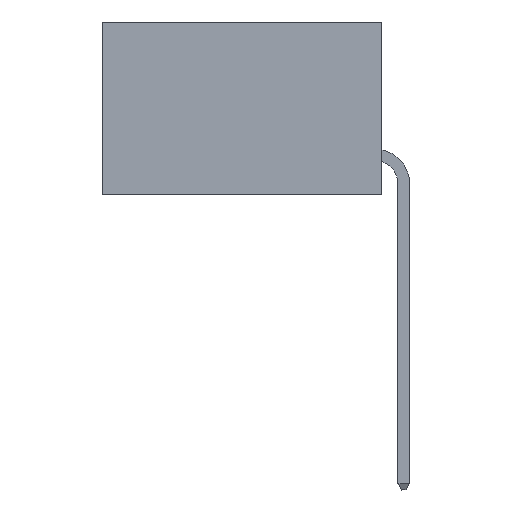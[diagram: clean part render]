
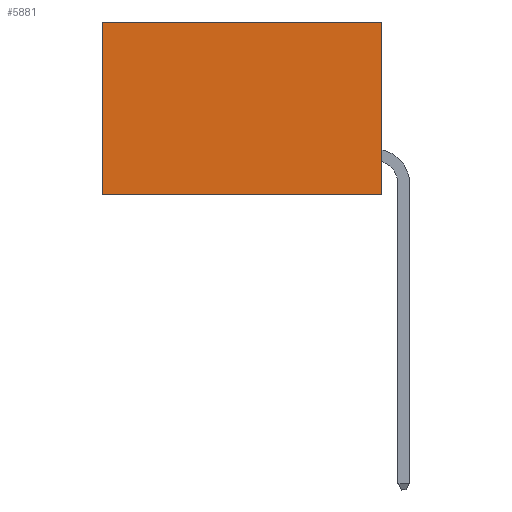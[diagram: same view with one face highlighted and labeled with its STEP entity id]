
A CAD part, left-side view. The second image highlights one B-rep face of the part: STEP entity #5881.
In plain terms, the highlighted planar face has unit normal (-1, 0, 0).
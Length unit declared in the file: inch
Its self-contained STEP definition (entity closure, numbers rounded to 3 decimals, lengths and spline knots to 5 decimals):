
#321 = EDGE_CURVE ( 'NONE', #15729, #2210, #14465, .T. ) ;
#1019 = VERTEX_POINT ( 'NONE', #22329 ) ;
#1737 = CARTESIAN_POINT ( 'NONE',  ( 0.2875, 0.6, -0.37 ) ) ;
#2210 = VERTEX_POINT ( 'NONE', #9588 ) ;
#4248 = EDGE_CURVE ( 'NONE', #2210, #4599, #11331, .T. ) ;
#4437 = PLANE ( 'NONE',  #33246 ) ;
#4599 = VERTEX_POINT ( 'NONE', #1737 ) ;
#4905 = VECTOR ( 'NONE', #11310, 39.37008 ) ;
#5881 = ADVANCED_FACE ( 'NONE', ( #37400 ), #4437, .F. ) ;
#7510 = DIRECTION ( 'NONE',  ( 1., 0., 0. ) ) ;
#7844 = VECTOR ( 'NONE', #12053, 39.37008 ) ;
#9588 = CARTESIAN_POINT ( 'NONE',  ( 0.2875, 0., -0.37 ) ) ;
#10782 = CARTESIAN_POINT ( 'NONE',  ( 0.2875, 0., 0. ) ) ;
#10983 = CARTESIAN_POINT ( 'NONE',  ( 0.2875, 0.6, 0. ) ) ;
#11310 = DIRECTION ( 'NONE',  ( 0., 1., 0. ) ) ;
#11331 = LINE ( 'NONE', #11595, #25569 ) ;
#11595 = CARTESIAN_POINT ( 'NONE',  ( 0.2875, 0., -0.37 ) ) ;
#12053 = DIRECTION ( 'NONE',  ( 0., 0., -1. ) ) ;
#14465 = LINE ( 'NONE', #30299, #7844 ) ;
#14658 = DIRECTION ( 'NONE',  ( 0., 1., 0. ) ) ;
#15729 = VERTEX_POINT ( 'NONE', #35232 ) ;
#16946 = DIRECTION ( 'NONE',  ( 0., 0., -1. ) ) ;
#18547 = ORIENTED_EDGE ( 'NONE', *, *, #22920, .T. ) ;
#19754 = CARTESIAN_POINT ( 'NONE',  ( 0.2875, 0., 0. ) ) ;
#22329 = CARTESIAN_POINT ( 'NONE',  ( 0.2875, 0.6, 0. ) ) ;
#22920 = EDGE_CURVE ( 'NONE', #1019, #4599, #33536, .T. ) ;
#23930 = LINE ( 'NONE', #10782, #4905 ) ;
#25569 = VECTOR ( 'NONE', #14658, 39.37008 ) ;
#29267 = ORIENTED_EDGE ( 'NONE', *, *, #4248, .F. ) ;
#30299 = CARTESIAN_POINT ( 'NONE',  ( 0.2875, 0., 0. ) ) ;
#32159 = DIRECTION ( 'NONE',  ( 0., 0., -1. ) ) ;
#32583 = VECTOR ( 'NONE', #32159, 39.37008 ) ;
#33246 = AXIS2_PLACEMENT_3D ( 'NONE', #19754, #7510, #16946 ) ;
#33536 = LINE ( 'NONE', #10983, #32583 ) ;
#34425 = ORIENTED_EDGE ( 'NONE', *, *, #321, .F. ) ;
#34855 = EDGE_LOOP ( 'NONE', ( #18547, #29267, #34425, #36736 ) ) ;
#35232 = CARTESIAN_POINT ( 'NONE',  ( 0.2875, 0., 0. ) ) ;
#36736 = ORIENTED_EDGE ( 'NONE', *, *, #38510, .T. ) ;
#37400 = FACE_OUTER_BOUND ( 'NONE', #34855, .T. ) ;
#38510 = EDGE_CURVE ( 'NONE', #15729, #1019, #23930, .T. ) ;
